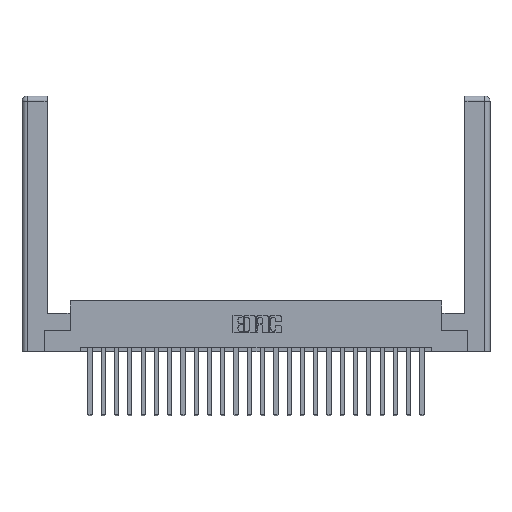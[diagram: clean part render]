
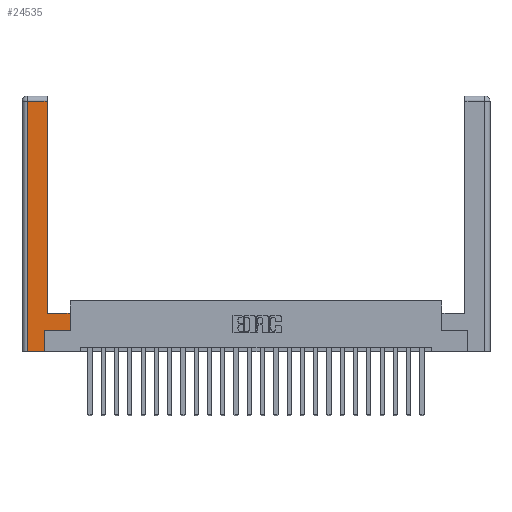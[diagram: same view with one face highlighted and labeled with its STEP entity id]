
A CAD part, top view. The second image highlights one B-rep face of the part: STEP entity #24535.
In plain terms, the highlighted planar face has unit normal (0, 0, 1).
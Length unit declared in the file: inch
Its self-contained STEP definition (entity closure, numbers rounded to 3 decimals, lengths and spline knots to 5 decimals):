
#41 = LINE ( 'NONE', #234, #3924 ) ;
#234 = CARTESIAN_POINT ( 'NONE',  ( 0.565, 0.245, 0. ) ) ;
#472 = CARTESIAN_POINT ( 'NONE',  ( 0.565, 0.45, 0. ) ) ;
#489 = DIRECTION ( 'NONE',  ( 0., -1., 0. ) ) ;
#556 = DIRECTION ( 'NONE',  ( 1., 0., 0. ) ) ;
#884 = EDGE_CURVE ( 'NONE', #21567, #15451, #4175, .T. ) ;
#1585 = LINE ( 'NONE', #472, #9339 ) ;
#2226 = CARTESIAN_POINT ( 'NONE',  ( 0.0615, 0., 0. ) ) ;
#2315 = DIRECTION ( 'NONE',  ( 0., 1., 0. ) ) ;
#2494 = EDGE_CURVE ( 'NONE', #9503, #21567, #7443, .T. ) ;
#2825 = VECTOR ( 'NONE', #2315, 39.37008 ) ;
#3459 = CARTESIAN_POINT ( 'NONE',  ( 0.295, 0.45, 0. ) ) ;
#3924 = VECTOR ( 'NONE', #21242, 39.37008 ) ;
#4175 = LINE ( 'NONE', #2226, #11284 ) ;
#4251 = AXIS2_PLACEMENT_3D ( 'NONE', #16964, #13018, #5569 ) ;
#4357 = VERTEX_POINT ( 'NONE', #20400 ) ;
#5569 = DIRECTION ( 'NONE',  ( -1., 0., 0. ) ) ;
#6099 = DIRECTION ( 'NONE',  ( -1., 0., 0. ) ) ;
#6451 = EDGE_CURVE ( 'NONE', #4357, #21949, #1585, .T. ) ;
#6722 = VERTEX_POINT ( 'NONE', #16198 ) ;
#7045 = LINE ( 'NONE', #8095, #21942 ) ;
#7443 = LINE ( 'NONE', #17385, #19666 ) ;
#7474 = LINE ( 'NONE', #11792, #18196 ) ;
#8095 = CARTESIAN_POINT ( 'NONE',  ( 0.295, 0.45, 0. ) ) ;
#8281 = ORIENTED_EDGE ( 'NONE', *, *, #19537, .T. ) ;
#8973 = VERTEX_POINT ( 'NONE', #3459 ) ;
#9307 = ORIENTED_EDGE ( 'NONE', *, *, #20000, .T. ) ;
#9339 = VECTOR ( 'NONE', #14413, 39.37008 ) ;
#9503 = VERTEX_POINT ( 'NONE', #24514 ) ;
#10166 = VECTOR ( 'NONE', #14680, 39.37008 ) ;
#10770 = ORIENTED_EDGE ( 'NONE', *, *, #884, .T. ) ;
#10842 = CARTESIAN_POINT ( 'NONE',  ( 0.265, 0.245, 0. ) ) ;
#11284 = VECTOR ( 'NONE', #489, 39.37008 ) ;
#11485 = CARTESIAN_POINT ( 'NONE',  ( 0.0615, 0., 0. ) ) ;
#11569 = ORIENTED_EDGE ( 'NONE', *, *, #19223, .T. ) ;
#11792 = CARTESIAN_POINT ( 'NONE',  ( 0.265, 0., 0. ) ) ;
#11867 = DIRECTION ( 'NONE',  ( -1., 0., 0. ) ) ;
#12677 = EDGE_CURVE ( 'NONE', #21949, #8973, #7045, .T. ) ;
#13018 = DIRECTION ( 'NONE',  ( 0., 0., -1. ) ) ;
#14413 = DIRECTION ( 'NONE',  ( 0., 1., 0. ) ) ;
#14680 = DIRECTION ( 'NONE',  ( 0., 1., 0. ) ) ;
#14903 = ORIENTED_EDGE ( 'NONE', *, *, #6451, .T. ) ;
#14955 = EDGE_LOOP ( 'NONE', ( #19812, #21182, #10770, #9307, #11569, #8281, #14903, #18727 ) ) ;
#15021 = PLANE ( 'NONE',  #4251 ) ;
#15451 = VERTEX_POINT ( 'NONE', #11485 ) ;
#15965 = CARTESIAN_POINT ( 'NONE',  ( 0.295, 3., 0. ) ) ;
#16198 = CARTESIAN_POINT ( 'NONE',  ( 0.265, 0., 0. ) ) ;
#16500 = EDGE_CURVE ( 'NONE', #8973, #9503, #17749, .T. ) ;
#16964 = CARTESIAN_POINT ( 'NONE',  ( 0., 0., 0. ) ) ;
#17385 = CARTESIAN_POINT ( 'NONE',  ( 0.0615, 2.94, 0. ) ) ;
#17749 = LINE ( 'NONE', #15965, #2825 ) ;
#18196 = VECTOR ( 'NONE', #556, 39.37008 ) ;
#18499 = CARTESIAN_POINT ( 'NONE',  ( 0.265, 0.245, 0. ) ) ;
#18727 = ORIENTED_EDGE ( 'NONE', *, *, #12677, .T. ) ;
#18786 = FACE_OUTER_BOUND ( 'NONE', #14955, .T. ) ;
#19101 = CARTESIAN_POINT ( 'NONE',  ( 0.565, 0.45, 0. ) ) ;
#19223 = EDGE_CURVE ( 'NONE', #6722, #21440, #23011, .T. ) ;
#19537 = EDGE_CURVE ( 'NONE', #21440, #4357, #41, .T. ) ;
#19666 = VECTOR ( 'NONE', #11867, 39.37008 ) ;
#19812 = ORIENTED_EDGE ( 'NONE', *, *, #16500, .T. ) ;
#20000 = EDGE_CURVE ( 'NONE', #15451, #6722, #7474, .T. ) ;
#20400 = CARTESIAN_POINT ( 'NONE',  ( 0.565, 0.245, 0. ) ) ;
#21182 = ORIENTED_EDGE ( 'NONE', *, *, #2494, .T. ) ;
#21242 = DIRECTION ( 'NONE',  ( 1., 0., 0. ) ) ;
#21440 = VERTEX_POINT ( 'NONE', #18499 ) ;
#21567 = VERTEX_POINT ( 'NONE', #24676 ) ;
#21942 = VECTOR ( 'NONE', #6099, 39.37008 ) ;
#21949 = VERTEX_POINT ( 'NONE', #19101 ) ;
#23011 = LINE ( 'NONE', #10842, #10166 ) ;
#24514 = CARTESIAN_POINT ( 'NONE',  ( 0.295, 2.94, 0. ) ) ;
#24535 = ADVANCED_FACE ( 'NONE', ( #18786 ), #15021, .F. ) ;
#24676 = CARTESIAN_POINT ( 'NONE',  ( 0.0615, 2.94, 0. ) ) ;
